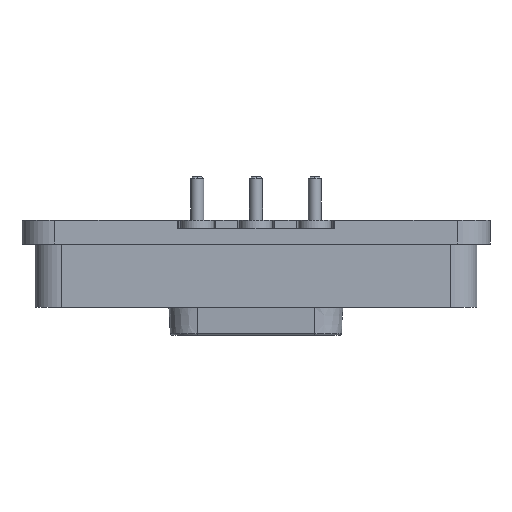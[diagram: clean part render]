
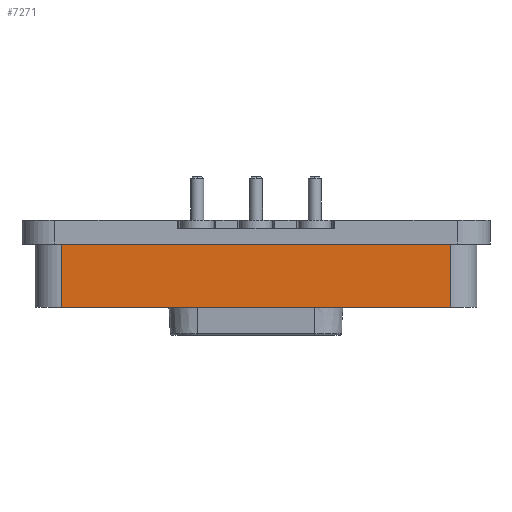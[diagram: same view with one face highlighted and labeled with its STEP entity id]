
A CAD part, left-side view. The second image highlights one B-rep face of the part: STEP entity #7271.
In plain terms, the highlighted planar face has unit normal (-1, 0, 0).
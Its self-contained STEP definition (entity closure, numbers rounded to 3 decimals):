
#489 = VECTOR ( 'NONE', #1887, 1000. ) ;
#1456 = DIRECTION ( 'NONE',  ( 0., 1., 0. ) ) ;
#1533 = DIRECTION ( 'NONE',  ( 0., 0., 1. ) ) ;
#1613 = ORIENTED_EDGE ( 'NONE', *, *, #3460, .F. ) ;
#1887 = DIRECTION ( 'NONE',  ( 0., 0., -1. ) ) ;
#2090 = FACE_OUTER_BOUND ( 'NONE', #2388, .T. ) ;
#2126 = CARTESIAN_POINT ( 'NONE',  ( -1.75, 8.95, 14.802 ) ) ;
#2164 = VECTOR ( 'NONE', #3530, 1000. ) ;
#2388 = EDGE_LOOP ( 'NONE', ( #5478, #5560, #1613, #3233 ) ) ;
#2966 = VECTOR ( 'NONE', #1456, 1000. ) ;
#3053 = VERTEX_POINT ( 'NONE', #6001 ) ;
#3233 = ORIENTED_EDGE ( 'NONE', *, *, #5423, .F. ) ;
#3274 = LINE ( 'NONE', #5183, #2966 ) ;
#3298 = DIRECTION ( 'NONE',  ( 0., -1., 0. ) ) ;
#3414 = AXIS2_PLACEMENT_3D ( 'NONE', #4606, #5051, #1533 ) ;
#3460 = EDGE_CURVE ( 'NONE', #3053, #7802, #3274, .T. ) ;
#3530 = DIRECTION ( 'NONE',  ( 0., 0., 1. ) ) ;
#4035 = LINE ( 'NONE', #2126, #5477 ) ;
#4350 = LINE ( 'NONE', #7440, #489 ) ;
#4462 = VERTEX_POINT ( 'NONE', #6937 ) ;
#4606 = CARTESIAN_POINT ( 'NONE',  ( -1.75, -10.15, 15.902 ) ) ;
#4930 = EDGE_CURVE ( 'NONE', #7802, #4462, #5503, .T. ) ;
#5051 = DIRECTION ( 'NONE',  ( -1., 0., 0. ) ) ;
#5183 = CARTESIAN_POINT ( 'NONE',  ( -1.75, -8.95, 11.902 ) ) ;
#5213 = PLANE ( 'NONE',  #3414 ) ;
#5423 = EDGE_CURVE ( 'NONE', #5872, #3053, #4350, .T. ) ;
#5477 = VECTOR ( 'NONE', #3298, 1000. ) ;
#5478 = ORIENTED_EDGE ( 'NONE', *, *, #6533, .F. ) ;
#5503 = LINE ( 'NONE', #7899, #2164 ) ;
#5560 = ORIENTED_EDGE ( 'NONE', *, *, #4930, .F. ) ;
#5872 = VERTEX_POINT ( 'NONE', #7412 ) ;
#5992 = CARTESIAN_POINT ( 'NONE',  ( -1.75, 8.95, 11.902 ) ) ;
#6001 = CARTESIAN_POINT ( 'NONE',  ( -1.75, -8.95, 11.902 ) ) ;
#6533 = EDGE_CURVE ( 'NONE', #4462, #5872, #4035, .T. ) ;
#6937 = CARTESIAN_POINT ( 'NONE',  ( -1.75, 8.95, 14.802 ) ) ;
#7271 = ADVANCED_FACE ( 'NONE', ( #2090 ), #5213, .T. ) ;
#7412 = CARTESIAN_POINT ( 'NONE',  ( -1.75, -8.95, 14.802 ) ) ;
#7440 = CARTESIAN_POINT ( 'NONE',  ( -1.75, -8.95, 14.802 ) ) ;
#7802 = VERTEX_POINT ( 'NONE', #5992 ) ;
#7899 = CARTESIAN_POINT ( 'NONE',  ( -1.75, 8.95, 11.902 ) ) ;
